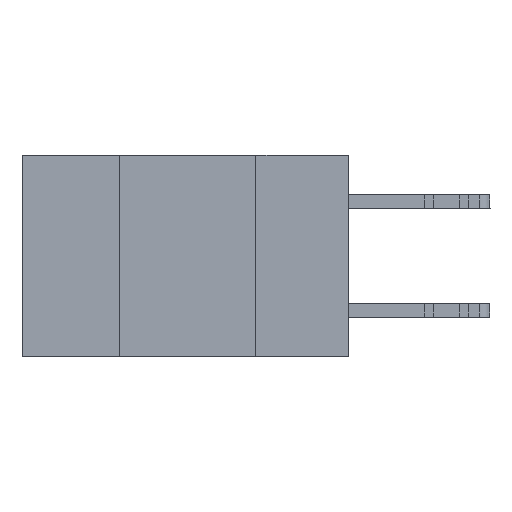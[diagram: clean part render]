
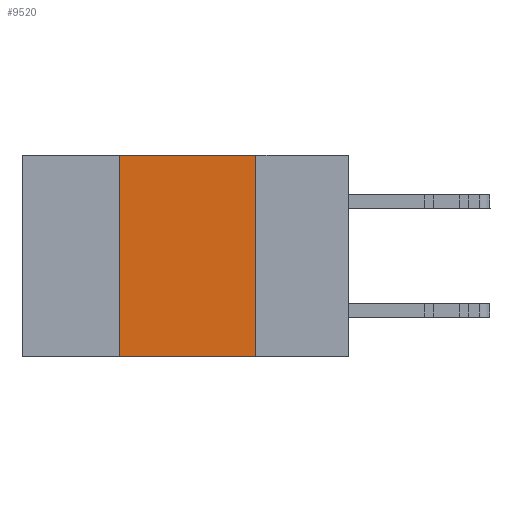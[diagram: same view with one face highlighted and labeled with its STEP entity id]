
A CAD part, left-side view. The second image highlights one B-rep face of the part: STEP entity #9520.
In plain terms, the highlighted planar face has unit normal (-1, 0, 0).
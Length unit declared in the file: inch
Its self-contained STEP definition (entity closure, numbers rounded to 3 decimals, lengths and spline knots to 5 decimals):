
#5 = CARTESIAN_POINT ( 'NONE',  ( 0., 0.17, -0.37 ) ) ;
#135 = EDGE_CURVE ( 'NONE', #19040, #18781, #5711, .T. ) ;
#474 = DIRECTION ( 'NONE',  ( 0., -1., 0. ) ) ;
#656 = VERTEX_POINT ( 'NONE', #5 ) ;
#701 = VECTOR ( 'NONE', #2738, 39.37008 ) ;
#1323 = AXIS2_PLACEMENT_3D ( 'NONE', #29273, #4032, #1855 ) ;
#1508 = ORIENTED_EDGE ( 'NONE', *, *, #135, .F. ) ;
#1855 = DIRECTION ( 'NONE',  ( 0., 0., -1. ) ) ;
#2080 = CARTESIAN_POINT ( 'NONE',  ( 0., 0.6, -0.37 ) ) ;
#2392 = FACE_OUTER_BOUND ( 'NONE', #24766, .T. ) ;
#2738 = DIRECTION ( 'NONE',  ( 0., 0., 1. ) ) ;
#3388 = LINE ( 'NONE', #7273, #25774 ) ;
#4032 = DIRECTION ( 'NONE',  ( 1., 0., 0. ) ) ;
#4332 = CARTESIAN_POINT ( 'NONE',  ( 0., 0.17, 0. ) ) ;
#4341 = PLANE ( 'NONE',  #1323 ) ;
#4470 = CARTESIAN_POINT ( 'NONE',  ( 0., 0.42, 0. ) ) ;
#5711 = LINE ( 'NONE', #8885, #701 ) ;
#7273 = CARTESIAN_POINT ( 'NONE',  ( 0., 0.6, 0. ) ) ;
#8690 = EDGE_CURVE ( 'NONE', #13378, #656, #20563, .T. ) ;
#8885 = CARTESIAN_POINT ( 'NONE',  ( 0., 0.42, 0. ) ) ;
#9077 = VECTOR ( 'NONE', #22457, 39.37008 ) ;
#9520 = ADVANCED_FACE ( 'NONE', ( #2392 ), #4341, .F. ) ;
#11535 = CARTESIAN_POINT ( 'NONE',  ( 0., 0.17, 0. ) ) ;
#13378 = VERTEX_POINT ( 'NONE', #4332 ) ;
#14093 = ORIENTED_EDGE ( 'NONE', *, *, #8690, .F. ) ;
#18764 = EDGE_CURVE ( 'NONE', #19040, #656, #21399, .T. ) ;
#18781 = VERTEX_POINT ( 'NONE', #4470 ) ;
#19040 = VERTEX_POINT ( 'NONE', #27871 ) ;
#19912 = ORIENTED_EDGE ( 'NONE', *, *, #18764, .T. ) ;
#20563 = LINE ( 'NONE', #11535, #24829 ) ;
#21399 = LINE ( 'NONE', #2080, #9077 ) ;
#22457 = DIRECTION ( 'NONE',  ( 0., -1., 0. ) ) ;
#22869 = DIRECTION ( 'NONE',  ( 0., 0., -1. ) ) ;
#24766 = EDGE_LOOP ( 'NONE', ( #14093, #25395, #1508, #19912 ) ) ;
#24829 = VECTOR ( 'NONE', #22869, 39.37008 ) ;
#25395 = ORIENTED_EDGE ( 'NONE', *, *, #28021, .F. ) ;
#25774 = VECTOR ( 'NONE', #474, 39.37008 ) ;
#27871 = CARTESIAN_POINT ( 'NONE',  ( 0., 0.42, -0.37 ) ) ;
#28021 = EDGE_CURVE ( 'NONE', #18781, #13378, #3388, .T. ) ;
#29273 = CARTESIAN_POINT ( 'NONE',  ( 0., 0.6, 0. ) ) ;
